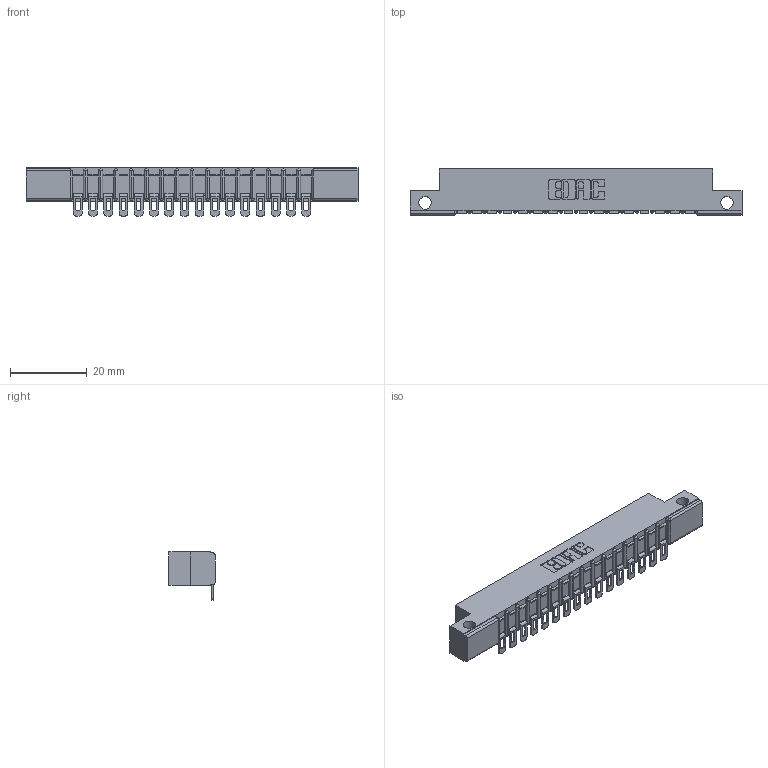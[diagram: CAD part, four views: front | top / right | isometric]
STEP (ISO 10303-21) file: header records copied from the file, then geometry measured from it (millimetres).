
FILE_DESCRIPTION (( 'STEP AP203' ), '1' );
FILE_NAME ('307-016-454-112.STEP', '2020-09-25T20:17:32', ( '' ), ( '' ), 'SwSTEP 2.0', 'SolidWorks 2020', '' );
FILE_SCHEMA (( 'CONFIG_CONTROL_DESIGN' ));
Length unit declared in the file: inch
Products named in the file (3): 307 Part_.128 Dia Side Mounting Holes; 307-016-454-112; 307-290-002_554
Assembly tree (17 placements, depth 2):
  307-016-454-112
    307 Part_.128 Dia Side Mounting Holes
    307-290-002_554  x16
Bounding box: 86.41 x 12.01 x 12.52 mm (x, y, z)
Volume: 5631.4 mm3; surface area: 9837.2 mm2
Topology: 17 solids, 17 shells, 1431 faces, 4371 edges, 2866 vertices
Faces by surface type: plane 806, cylinder 591, sphere 34
Entity records: 17889 total; most frequent: CARTESIAN_POINT 3014, ORIENTED_EDGE 3004, DIRECTION 2946, EDGE_CURVE 1502, VECTOR 1130, LINE 1130, VERTEX_POINT 976, AXIS2_PLACEMENT_3D 908
